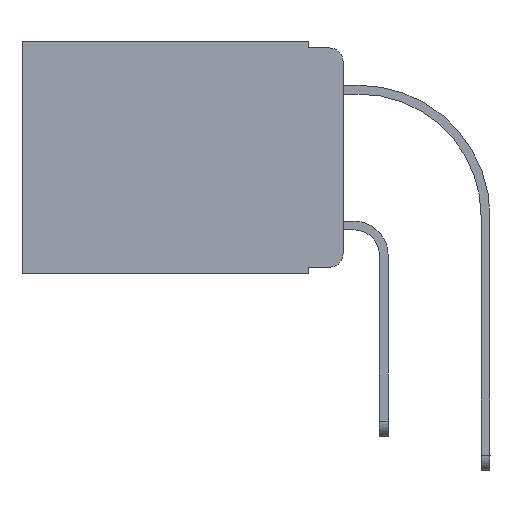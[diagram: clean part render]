
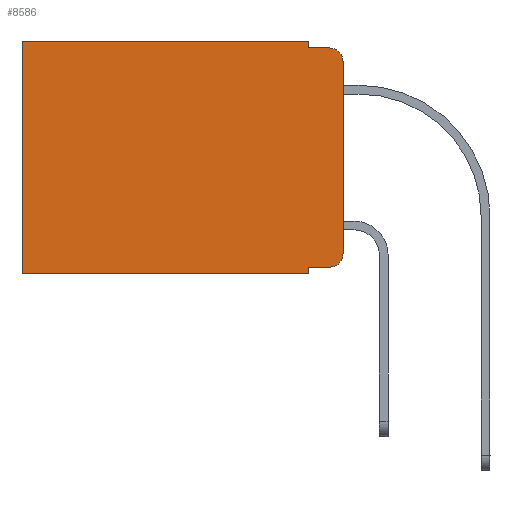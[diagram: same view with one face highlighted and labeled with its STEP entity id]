
A CAD part, left-side view. The second image highlights one B-rep face of the part: STEP entity #8586.
In plain terms, the highlighted planar face has unit normal (-1, 0, 0).
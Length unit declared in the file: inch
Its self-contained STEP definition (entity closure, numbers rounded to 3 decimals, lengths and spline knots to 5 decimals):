
#469 = CARTESIAN_POINT ( 'NONE',  ( 0.298, 0.473, 0. ) ) ;
#1200 = CARTESIAN_POINT ( 'NONE',  ( 0.298, 0.051, -0.01 ) ) ;
#1354 = LINE ( 'NONE', #7309, #18976 ) ;
#1461 = CARTESIAN_POINT ( 'NONE',  ( 0.298, 0.02, -0.03 ) ) ;
#1756 = VERTEX_POINT ( 'NONE', #14920 ) ;
#1767 = CARTESIAN_POINT ( 'NONE',  ( 0.298, 0., 0. ) ) ;
#2150 = VERTEX_POINT ( 'NONE', #7320 ) ;
#2261 = CARTESIAN_POINT ( 'NONE',  ( 0.298, 0., -0.343 ) ) ;
#2388 = EDGE_CURVE ( 'NONE', #4259, #2678, #9577, .T. ) ;
#2409 = CIRCLE ( 'NONE', #13669, 0.02 ) ;
#2465 = LINE ( 'NONE', #6763, #5568 ) ;
#2478 = LINE ( 'NONE', #4290, #14458 ) ;
#2647 = CARTESIAN_POINT ( 'NONE',  ( 0.298, 0.02, -0.313 ) ) ;
#2678 = VERTEX_POINT ( 'NONE', #469 ) ;
#2944 = DIRECTION ( 'NONE',  ( 0., -1., 0. ) ) ;
#3066 = VERTEX_POINT ( 'NONE', #6126 ) ;
#3638 = ORIENTED_EDGE ( 'NONE', *, *, #7614, .F. ) ;
#3670 = LINE ( 'NONE', #14159, #4342 ) ;
#4173 = AXIS2_PLACEMENT_3D ( 'NONE', #1461, #11736, #14797 ) ;
#4259 = VERTEX_POINT ( 'NONE', #8677 ) ;
#4290 = CARTESIAN_POINT ( 'NONE',  ( 0.298, 0.051, 0. ) ) ;
#4342 = VECTOR ( 'NONE', #7958, 39.37008 ) ;
#4791 = ORIENTED_EDGE ( 'NONE', *, *, #6348, .T. ) ;
#5089 = LINE ( 'NONE', #2261, #17180 ) ;
#5328 = EDGE_CURVE ( 'NONE', #10945, #15953, #5886, .T. ) ;
#5568 = VECTOR ( 'NONE', #11283, 39.37008 ) ;
#5584 = DIRECTION ( 'NONE',  ( 0., 0., -1. ) ) ;
#5886 = LINE ( 'NONE', #14923, #14898 ) ;
#6126 = CARTESIAN_POINT ( 'NONE',  ( 0.298, 0.473, -0.343 ) ) ;
#6348 = EDGE_CURVE ( 'NONE', #2678, #3066, #3670, .T. ) ;
#6451 = DIRECTION ( 'NONE',  ( 0., 1., 0. ) ) ;
#6763 = CARTESIAN_POINT ( 'NONE',  ( 0.298, 0.051, 0. ) ) ;
#7309 = CARTESIAN_POINT ( 'NONE',  ( 0.298, 0., 0. ) ) ;
#7320 = CARTESIAN_POINT ( 'NONE',  ( 0.298, 0.02, -0.333 ) ) ;
#7377 = VECTOR ( 'NONE', #16108, 39.37008 ) ;
#7614 = EDGE_CURVE ( 'NONE', #10232, #1756, #1354, .T. ) ;
#7626 = PLANE ( 'NONE',  #8644 ) ;
#7770 = VERTEX_POINT ( 'NONE', #18012 ) ;
#7958 = DIRECTION ( 'NONE',  ( 0., 0., -1. ) ) ;
#8027 = FACE_OUTER_BOUND ( 'NONE', #11382, .T. ) ;
#8234 = CARTESIAN_POINT ( 'NONE',  ( 0.298, 0.02, -0.01 ) ) ;
#8586 = ADVANCED_FACE ( 'NONE', ( #8027 ), #7626, .F. ) ;
#8644 = AXIS2_PLACEMENT_3D ( 'NONE', #1767, #13919, #18243 ) ;
#8677 = CARTESIAN_POINT ( 'NONE',  ( 0.298, 0.051, 0. ) ) ;
#9577 = LINE ( 'NONE', #13908, #10475 ) ;
#9712 = EDGE_CURVE ( 'NONE', #15993, #2150, #11602, .T. ) ;
#10211 = EDGE_CURVE ( 'NONE', #15993, #7770, #2478, .T. ) ;
#10232 = VERTEX_POINT ( 'NONE', #14791 ) ;
#10264 = DIRECTION ( 'NONE',  ( 0., 0., -1. ) ) ;
#10475 = VECTOR ( 'NONE', #6451, 39.37008 ) ;
#10924 = ORIENTED_EDGE ( 'NONE', *, *, #9712, .T. ) ;
#10945 = VERTEX_POINT ( 'NONE', #1200 ) ;
#11283 = DIRECTION ( 'NONE',  ( 0., 0., -1. ) ) ;
#11382 = EDGE_LOOP ( 'NONE', ( #3638, #12052, #12355, #11654, #18256, #4791, #14939, #13245, #10924, #14808 ) ) ;
#11602 = LINE ( 'NONE', #19353, #7377 ) ;
#11654 = ORIENTED_EDGE ( 'NONE', *, *, #15941, .F. ) ;
#11736 = DIRECTION ( 'NONE',  ( -1., 0., 0. ) ) ;
#12052 = ORIENTED_EDGE ( 'NONE', *, *, #12678, .T. ) ;
#12355 = ORIENTED_EDGE ( 'NONE', *, *, #5328, .F. ) ;
#12678 = EDGE_CURVE ( 'NONE', #10232, #15953, #18909, .T. ) ;
#13245 = ORIENTED_EDGE ( 'NONE', *, *, #10211, .F. ) ;
#13669 = AXIS2_PLACEMENT_3D ( 'NONE', #2647, #14717, #5584 ) ;
#13908 = CARTESIAN_POINT ( 'NONE',  ( 0.298, 0., 0. ) ) ;
#13919 = DIRECTION ( 'NONE',  ( 1., 0., 0. ) ) ;
#14159 = CARTESIAN_POINT ( 'NONE',  ( 0.298, 0.473, 0. ) ) ;
#14331 = DIRECTION ( 'NONE',  ( 0., 1., 0. ) ) ;
#14458 = VECTOR ( 'NONE', #10264, 39.37008 ) ;
#14717 = DIRECTION ( 'NONE',  ( -1., 0., 0. ) ) ;
#14791 = CARTESIAN_POINT ( 'NONE',  ( 0.298, 0., -0.03 ) ) ;
#14797 = DIRECTION ( 'NONE',  ( 0., 0., -1. ) ) ;
#14808 = ORIENTED_EDGE ( 'NONE', *, *, #16067, .T. ) ;
#14898 = VECTOR ( 'NONE', #2944, 39.37008 ) ;
#14920 = CARTESIAN_POINT ( 'NONE',  ( 0.298, 0., -0.313 ) ) ;
#14923 = CARTESIAN_POINT ( 'NONE',  ( 0.298, 0.051, -0.01 ) ) ;
#14939 = ORIENTED_EDGE ( 'NONE', *, *, #15881, .F. ) ;
#15881 = EDGE_CURVE ( 'NONE', #7770, #3066, #5089, .T. ) ;
#15941 = EDGE_CURVE ( 'NONE', #4259, #10945, #2465, .T. ) ;
#15953 = VERTEX_POINT ( 'NONE', #8234 ) ;
#15993 = VERTEX_POINT ( 'NONE', #17747 ) ;
#16062 = DIRECTION ( 'NONE',  ( 0., 0., -1. ) ) ;
#16067 = EDGE_CURVE ( 'NONE', #2150, #1756, #2409, .T. ) ;
#16108 = DIRECTION ( 'NONE',  ( 0., -1., 0. ) ) ;
#17180 = VECTOR ( 'NONE', #14331, 39.37008 ) ;
#17747 = CARTESIAN_POINT ( 'NONE',  ( 0.298, 0.051, -0.333 ) ) ;
#18012 = CARTESIAN_POINT ( 'NONE',  ( 0.298, 0.051, -0.343 ) ) ;
#18243 = DIRECTION ( 'NONE',  ( 0., 0., -1. ) ) ;
#18256 = ORIENTED_EDGE ( 'NONE', *, *, #2388, .T. ) ;
#18909 = CIRCLE ( 'NONE', #4173, 0.02 ) ;
#18976 = VECTOR ( 'NONE', #16062, 39.37008 ) ;
#19353 = CARTESIAN_POINT ( 'NONE',  ( 0.298, 0.051, -0.333 ) ) ;
